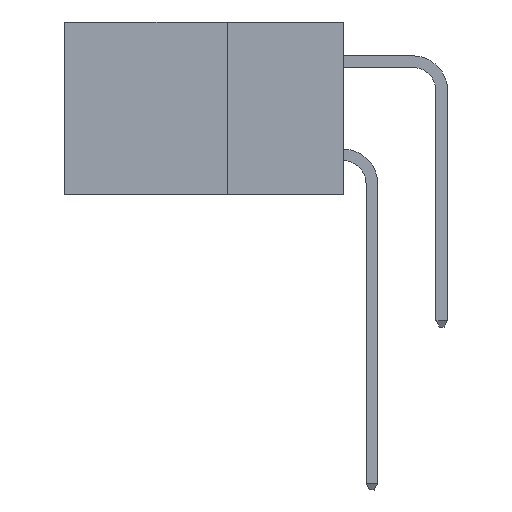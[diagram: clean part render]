
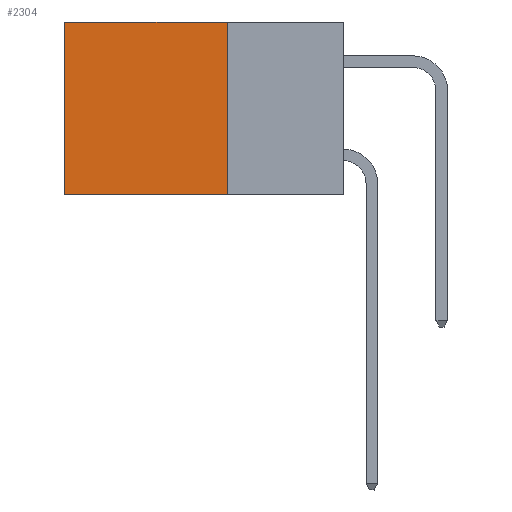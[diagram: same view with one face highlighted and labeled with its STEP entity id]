
A CAD part, left-side view. The second image highlights one B-rep face of the part: STEP entity #2304.
In plain terms, the highlighted planar face has unit normal (-1, 0, 0).
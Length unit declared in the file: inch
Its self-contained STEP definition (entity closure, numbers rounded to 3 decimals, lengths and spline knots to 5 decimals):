
#588 = PLANE ( 'NONE',  #1629 ) ;
#967 = VERTEX_POINT ( 'NONE', #11477 ) ;
#1125 = EDGE_CURVE ( 'NONE', #17832, #10407, #5480, .T. ) ;
#1397 = CARTESIAN_POINT ( 'NONE',  ( 0.298, 0.25, 0. ) ) ;
#1629 = AXIS2_PLACEMENT_3D ( 'NONE', #28274, #20804, #30799 ) ;
#2304 = ADVANCED_FACE ( 'NONE', ( #29653 ), #588, .F. ) ;
#2724 = DIRECTION ( 'NONE',  ( 0., 1., 0. ) ) ;
#2945 = ORIENTED_EDGE ( 'NONE', *, *, #18377, .T. ) ;
#3088 = VECTOR ( 'NONE', #2724, 39.37008 ) ;
#3880 = LINE ( 'NONE', #30634, #3088 ) ;
#5146 = EDGE_CURVE ( 'NONE', #967, #10407, #20252, .T. ) ;
#5310 = CARTESIAN_POINT ( 'NONE',  ( 0.298, 0.25, 0. ) ) ;
#5480 = LINE ( 'NONE', #12239, #31308 ) ;
#9505 = EDGE_LOOP ( 'NONE', ( #26442, #25015, #23098, #2945 ) ) ;
#9714 = VECTOR ( 'NONE', #19556, 39.37008 ) ;
#10027 = CARTESIAN_POINT ( 'NONE',  ( 0.298, 0.6, -0.37 ) ) ;
#10407 = VERTEX_POINT ( 'NONE', #10027 ) ;
#11184 = CARTESIAN_POINT ( 'NONE',  ( 0.298, 0.25, -0.37 ) ) ;
#11477 = CARTESIAN_POINT ( 'NONE',  ( 0.298, 0.6, 0. ) ) ;
#12239 = CARTESIAN_POINT ( 'NONE',  ( 0.298, 0.25, -0.37 ) ) ;
#17832 = VERTEX_POINT ( 'NONE', #11184 ) ;
#18377 = EDGE_CURVE ( 'NONE', #25092, #967, #3880, .T. ) ;
#19556 = DIRECTION ( 'NONE',  ( 0., 0., -1. ) ) ;
#20252 = LINE ( 'NONE', #24633, #9714 ) ;
#20804 = DIRECTION ( 'NONE',  ( 1., 0., 0. ) ) ;
#23098 = ORIENTED_EDGE ( 'NONE', *, *, #27602, .F. ) ;
#23236 = DIRECTION ( 'NONE',  ( 0., 0., -1. ) ) ;
#24003 = LINE ( 'NONE', #5310, #31043 ) ;
#24633 = CARTESIAN_POINT ( 'NONE',  ( 0.298, 0.6, 0. ) ) ;
#25015 = ORIENTED_EDGE ( 'NONE', *, *, #1125, .F. ) ;
#25092 = VERTEX_POINT ( 'NONE', #1397 ) ;
#26442 = ORIENTED_EDGE ( 'NONE', *, *, #5146, .T. ) ;
#27602 = EDGE_CURVE ( 'NONE', #25092, #17832, #24003, .T. ) ;
#28274 = CARTESIAN_POINT ( 'NONE',  ( 0.298, 0.25, 0. ) ) ;
#29653 = FACE_OUTER_BOUND ( 'NONE', #9505, .T. ) ;
#30634 = CARTESIAN_POINT ( 'NONE',  ( 0.298, 0.25, 0. ) ) ;
#30799 = DIRECTION ( 'NONE',  ( 0., 0., -1. ) ) ;
#31043 = VECTOR ( 'NONE', #23236, 39.37008 ) ;
#31308 = VECTOR ( 'NONE', #32325, 39.37008 ) ;
#32325 = DIRECTION ( 'NONE',  ( 0., 1., 0. ) ) ;
